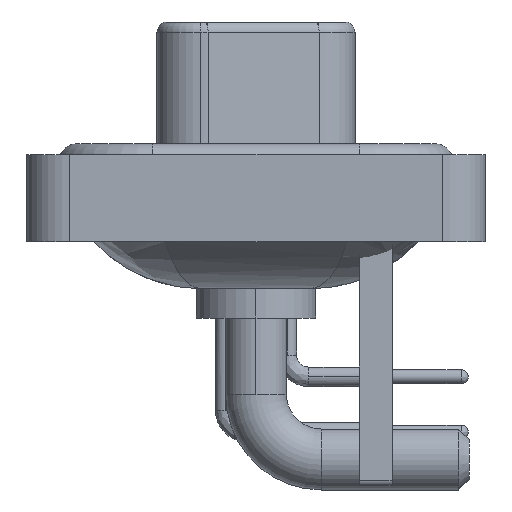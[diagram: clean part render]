
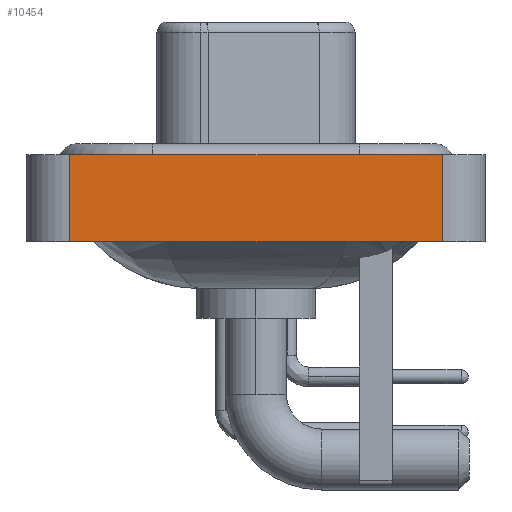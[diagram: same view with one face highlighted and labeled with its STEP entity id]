
A CAD part, left-side view. The second image highlights one B-rep face of the part: STEP entity #10454.
In plain terms, the highlighted planar face has unit normal (-1, 0, 0).
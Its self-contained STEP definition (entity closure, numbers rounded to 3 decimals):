
#261 = EDGE_CURVE ( 'NONE', #13168, #27443, #26440, .T. ) ;
#458 = EDGE_LOOP ( 'NONE', ( #6869, #21520, #21866, #14905 ) ) ;
#1147 = VECTOR ( 'NONE', #20918, 1000. ) ;
#2052 = LINE ( 'NONE', #17869, #1147 ) ;
#6869 = ORIENTED_EDGE ( 'NONE', *, *, #28927, .T. ) ;
#7088 = VECTOR ( 'NONE', #13327, 1000. ) ;
#7185 = CARTESIAN_POINT ( 'NONE',  ( -7.35, -8.55, -3.6 ) ) ;
#7794 = LINE ( 'NONE', #23894, #15684 ) ;
#9115 = DIRECTION ( 'NONE',  ( 0., -1., 0. ) ) ;
#10454 = ADVANCED_FACE ( 'NONE', ( #13135 ), #11067, .T. ) ;
#11067 = PLANE ( 'NONE',  #20161 ) ;
#11340 = LINE ( 'NONE', #20348, #20194 ) ;
#12103 = VERTEX_POINT ( 'NONE', #19988 ) ;
#12610 = VERTEX_POINT ( 'NONE', #7185 ) ;
#13135 = FACE_OUTER_BOUND ( 'NONE', #458, .T. ) ;
#13168 = VERTEX_POINT ( 'NONE', #24286 ) ;
#13327 = DIRECTION ( 'NONE',  ( 0., 0., 1. ) ) ;
#13421 = CARTESIAN_POINT ( 'NONE',  ( -7.35, 8.55, 0.4 ) ) ;
#14905 = ORIENTED_EDGE ( 'NONE', *, *, #15701, .T. ) ;
#15645 = DIRECTION ( 'NONE',  ( 0., 0., 1. ) ) ;
#15684 = VECTOR ( 'NONE', #19172, 1000. ) ;
#15701 = EDGE_CURVE ( 'NONE', #13168, #12610, #2052, .T. ) ;
#17851 = CARTESIAN_POINT ( 'NONE',  ( -7.35, -8.55, -3.6 ) ) ;
#17869 = CARTESIAN_POINT ( 'NONE',  ( -7.35, -8.55, -3.6 ) ) ;
#19172 = DIRECTION ( 'NONE',  ( 0., 0., 1. ) ) ;
#19691 = CARTESIAN_POINT ( 'NONE',  ( -7.35, 8.55, -3.6 ) ) ;
#19988 = CARTESIAN_POINT ( 'NONE',  ( -7.35, -8.55, 0.4 ) ) ;
#20161 = AXIS2_PLACEMENT_3D ( 'NONE', #17851, #26827, #15645 ) ;
#20194 = VECTOR ( 'NONE', #9115, 1000. ) ;
#20348 = CARTESIAN_POINT ( 'NONE',  ( -7.35, -8.55, 0.4 ) ) ;
#20918 = DIRECTION ( 'NONE',  ( 0., -1., 0. ) ) ;
#21520 = ORIENTED_EDGE ( 'NONE', *, *, #26287, .F. ) ;
#21866 = ORIENTED_EDGE ( 'NONE', *, *, #261, .F. ) ;
#23894 = CARTESIAN_POINT ( 'NONE',  ( -7.35, -8.55, -3.6 ) ) ;
#24286 = CARTESIAN_POINT ( 'NONE',  ( -7.35, 8.55, -3.6 ) ) ;
#26287 = EDGE_CURVE ( 'NONE', #27443, #12103, #11340, .T. ) ;
#26440 = LINE ( 'NONE', #19691, #7088 ) ;
#26827 = DIRECTION ( 'NONE',  ( -1., 0., 0. ) ) ;
#27443 = VERTEX_POINT ( 'NONE', #13421 ) ;
#28927 = EDGE_CURVE ( 'NONE', #12610, #12103, #7794, .T. ) ;
